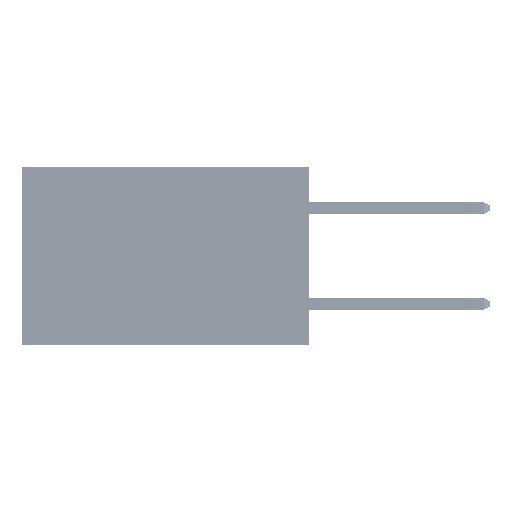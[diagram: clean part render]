
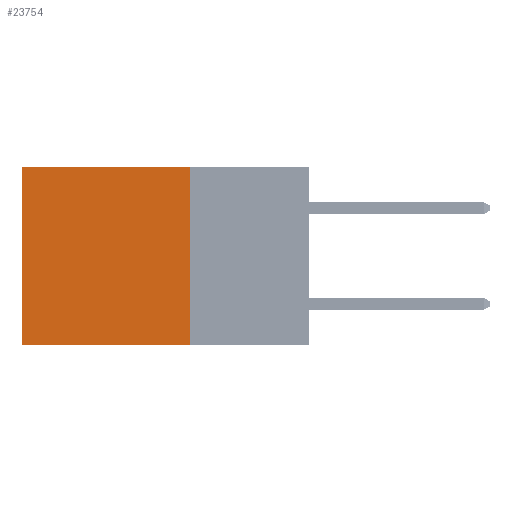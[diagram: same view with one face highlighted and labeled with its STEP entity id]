
A CAD part, left-side view. The second image highlights one B-rep face of the part: STEP entity #23754.
In plain terms, the highlighted planar face has unit normal (-1, 0, 0).
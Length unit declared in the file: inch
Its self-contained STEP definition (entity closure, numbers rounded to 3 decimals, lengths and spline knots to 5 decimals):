
#2120 = EDGE_CURVE ( 'NONE', #5173, #30120, #6461, .T. ) ;
#2500 = DIRECTION ( 'NONE',  ( 0., 0., -1. ) ) ;
#4807 = ORIENTED_EDGE ( 'NONE', *, *, #22681, .T. ) ;
#5173 = VERTEX_POINT ( 'NONE', #29927 ) ;
#6220 = FACE_OUTER_BOUND ( 'NONE', #51271, .T. ) ;
#6461 = LINE ( 'NONE', #22620, #43012 ) ;
#6821 = EDGE_CURVE ( 'NONE', #5173, #10785, #20381, .T. ) ;
#8543 = ORIENTED_EDGE ( 'NONE', *, *, #2120, .T. ) ;
#10785 = VERTEX_POINT ( 'NONE', #31459 ) ;
#12993 = VERTEX_POINT ( 'NONE', #44126 ) ;
#20263 = ORIENTED_EDGE ( 'NONE', *, *, #49496, .F. ) ;
#20381 = LINE ( 'NONE', #43944, #50485 ) ;
#22620 = CARTESIAN_POINT ( 'NONE',  ( 0.2875, 0.25, 0. ) ) ;
#22681 = EDGE_CURVE ( 'NONE', #30120, #12993, #28424, .T. ) ;
#23754 = ADVANCED_FACE ( 'NONE', ( #6220 ), #34533, .F. ) ;
#24438 = VECTOR ( 'NONE', #27044, 39.37008 ) ;
#26589 = DIRECTION ( 'NONE',  ( 0., 1., 0. ) ) ;
#27044 = DIRECTION ( 'NONE',  ( 0., 1., 0. ) ) ;
#28169 = DIRECTION ( 'NONE',  ( 0., 0., -1. ) ) ;
#28424 = LINE ( 'NONE', #49039, #44071 ) ;
#29927 = CARTESIAN_POINT ( 'NONE',  ( 0.2875, 0.25, 0. ) ) ;
#30120 = VERTEX_POINT ( 'NONE', #51255 ) ;
#30337 = ORIENTED_EDGE ( 'NONE', *, *, #6821, .F. ) ;
#30569 = DIRECTION ( 'NONE',  ( 1., 0., 0. ) ) ;
#30613 = AXIS2_PLACEMENT_3D ( 'NONE', #50678, #30569, #2500 ) ;
#31459 = CARTESIAN_POINT ( 'NONE',  ( 0.2875, 0.25, -0.37 ) ) ;
#34533 = PLANE ( 'NONE',  #30613 ) ;
#36017 = CARTESIAN_POINT ( 'NONE',  ( 0.2875, 0.25, -0.37 ) ) ;
#36275 = LINE ( 'NONE', #36017, #24438 ) ;
#43012 = VECTOR ( 'NONE', #26589, 39.37008 ) ;
#43944 = CARTESIAN_POINT ( 'NONE',  ( 0.2875, 0.25, 0. ) ) ;
#44071 = VECTOR ( 'NONE', #28169, 39.37008 ) ;
#44126 = CARTESIAN_POINT ( 'NONE',  ( 0.2875, 0.6, -0.37 ) ) ;
#44978 = DIRECTION ( 'NONE',  ( 0., 0., -1. ) ) ;
#49039 = CARTESIAN_POINT ( 'NONE',  ( 0.2875, 0.6, 0. ) ) ;
#49496 = EDGE_CURVE ( 'NONE', #10785, #12993, #36275, .T. ) ;
#50485 = VECTOR ( 'NONE', #44978, 39.37008 ) ;
#50678 = CARTESIAN_POINT ( 'NONE',  ( 0.2875, 0.25, 0. ) ) ;
#51255 = CARTESIAN_POINT ( 'NONE',  ( 0.2875, 0.6, 0. ) ) ;
#51271 = EDGE_LOOP ( 'NONE', ( #4807, #20263, #30337, #8543 ) ) ;
